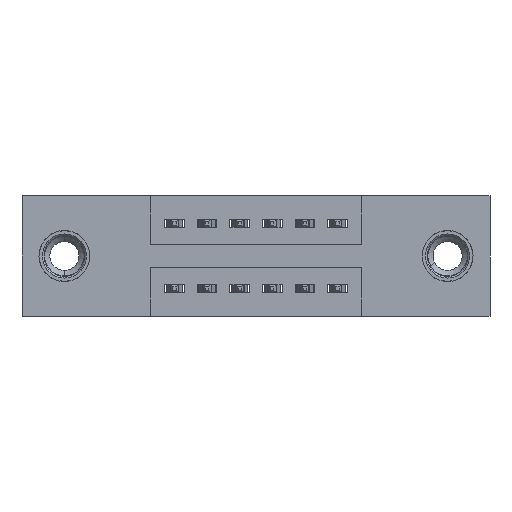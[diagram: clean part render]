
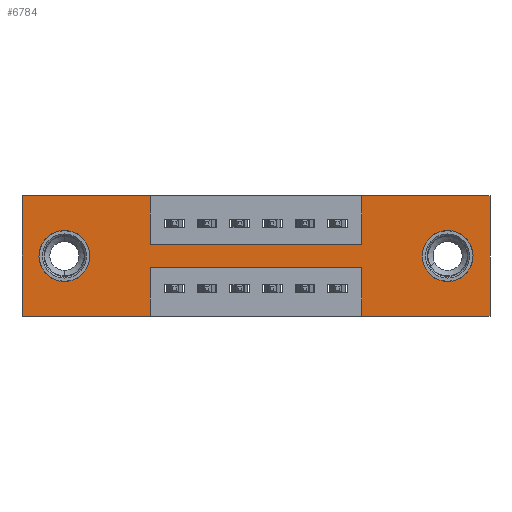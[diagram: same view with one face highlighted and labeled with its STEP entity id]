
A CAD part, front view. The second image highlights one B-rep face of the part: STEP entity #6784.
In plain terms, the highlighted planar face has unit normal (0, -1, 0).
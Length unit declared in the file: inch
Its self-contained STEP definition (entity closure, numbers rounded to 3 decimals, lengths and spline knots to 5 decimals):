
#75 = VERTEX_POINT ( 'NONE', #1648 ) ;
#120 = CARTESIAN_POINT ( 'NONE',  ( 0.13, 0., -0.185 ) ) ;
#124 = EDGE_CURVE ( 'NONE', #5131, #75, #7524, .T. ) ;
#136 = ORIENTED_EDGE ( 'NONE', *, *, #10163, .F. ) ;
#171 = VECTOR ( 'NONE', #3148, 39.37008 ) ;
#294 = LINE ( 'NONE', #9410, #8684 ) ;
#485 = DIRECTION ( 'NONE',  ( 1., 0., 0. ) ) ;
#491 = LINE ( 'NONE', #7586, #4763 ) ;
#546 = EDGE_CURVE ( 'NONE', #9718, #7218, #10677, .T. ) ;
#594 = VERTEX_POINT ( 'NONE', #8205 ) ;
#686 = AXIS2_PLACEMENT_3D ( 'NONE', #10744, #5892, #879 ) ;
#742 = EDGE_CURVE ( 'NONE', #75, #2618, #294, .T. ) ;
#811 = AXIS2_PLACEMENT_3D ( 'NONE', #6003, #996, #6815 ) ;
#876 = CIRCLE ( 'NONE', #9910, 0.078 ) ;
#879 = DIRECTION ( 'NONE',  ( 0., 0., 1. ) ) ;
#885 = PLANE ( 'NONE',  #5224 ) ;
#996 = DIRECTION ( 'NONE',  ( 0., 1., 0. ) ) ;
#1025 = DIRECTION ( 'NONE',  ( 0., 0., -1. ) ) ;
#1043 = DIRECTION ( 'NONE',  ( 0., 0., 1. ) ) ;
#1084 = CARTESIAN_POINT ( 'NONE',  ( 1.305, 0., -0.107 ) ) ;
#1213 = CARTESIAN_POINT ( 'NONE',  ( 0.3925, 0., 0. ) ) ;
#1319 = VERTEX_POINT ( 'NONE', #9587 ) ;
#1353 = EDGE_CURVE ( 'NONE', #5016, #7553, #8397, .T. ) ;
#1615 = VERTEX_POINT ( 'NONE', #6259 ) ;
#1645 = CARTESIAN_POINT ( 'NONE',  ( 1.0425, 0., 0. ) ) ;
#1648 = CARTESIAN_POINT ( 'NONE',  ( 0.3925, 0., -0.22 ) ) ;
#1689 = ORIENTED_EDGE ( 'NONE', *, *, #124, .F. ) ;
#1775 = DIRECTION ( 'NONE',  ( 0., 0., -1. ) ) ;
#1979 = VERTEX_POINT ( 'NONE', #8254 ) ;
#2053 = CARTESIAN_POINT ( 'NONE',  ( 1.305, 0., -0.263 ) ) ;
#2247 = ORIENTED_EDGE ( 'NONE', *, *, #9821, .F. ) ;
#2309 = VERTEX_POINT ( 'NONE', #7028 ) ;
#2618 = VERTEX_POINT ( 'NONE', #3358 ) ;
#2709 = CARTESIAN_POINT ( 'NONE',  ( 0.3925, 0., -0.15 ) ) ;
#2871 = FACE_BOUND ( 'NONE', #10533, .T. ) ;
#3089 = EDGE_LOOP ( 'NONE', ( #9894, #5834 ) ) ;
#3137 = ORIENTED_EDGE ( 'NONE', *, *, #1353, .T. ) ;
#3148 = DIRECTION ( 'NONE',  ( -1., 0., 0. ) ) ;
#3164 = VERTEX_POINT ( 'NONE', #8344 ) ;
#3282 = CARTESIAN_POINT ( 'NONE',  ( 1.435, 0., 0. ) ) ;
#3358 = CARTESIAN_POINT ( 'NONE',  ( 0.3925, 0., -0.37 ) ) ;
#3360 = CARTESIAN_POINT ( 'NONE',  ( 0.3925, 0., -0.22 ) ) ;
#3452 = EDGE_CURVE ( 'NONE', #1319, #3164, #8162, .T. ) ;
#3631 = EDGE_CURVE ( 'NONE', #2618, #2309, #4732, .T. ) ;
#3648 = CARTESIAN_POINT ( 'NONE',  ( 0.3925, 0., -0.15 ) ) ;
#3752 = VECTOR ( 'NONE', #9447, 39.37008 ) ;
#4158 = ORIENTED_EDGE ( 'NONE', *, *, #7450, .F. ) ;
#4180 = DIRECTION ( 'NONE',  ( 0., 0., -1. ) ) ;
#4237 = EDGE_LOOP ( 'NONE', ( #8005, #1689, #6103, #8256, #4158, #10658, #2247, #4429, #6604, #8795, #136, #4700 ) ) ;
#4297 = CARTESIAN_POINT ( 'NONE',  ( 1.305, 0., -0.185 ) ) ;
#4429 = ORIENTED_EDGE ( 'NONE', *, *, #9304, .F. ) ;
#4479 = EDGE_CURVE ( 'NONE', #1615, #1979, #5351, .T. ) ;
#4559 = VERTEX_POINT ( 'NONE', #2709 ) ;
#4600 = AXIS2_PLACEMENT_3D ( 'NONE', #4297, #8379, #8233 ) ;
#4700 = ORIENTED_EDGE ( 'NONE', *, *, #3631, .F. ) ;
#4732 = LINE ( 'NONE', #4815, #171 ) ;
#4763 = VECTOR ( 'NONE', #9213, 39.37008 ) ;
#4815 = CARTESIAN_POINT ( 'NONE',  ( 0., 0., -0.37 ) ) ;
#4956 = EDGE_CURVE ( 'NONE', #1979, #1615, #876, .T. ) ;
#5016 = VERTEX_POINT ( 'NONE', #1084 ) ;
#5131 = VERTEX_POINT ( 'NONE', #9504 ) ;
#5224 = AXIS2_PLACEMENT_3D ( 'NONE', #9161, #6718, #1775 ) ;
#5299 = FACE_BOUND ( 'NONE', #3089, .T. ) ;
#5351 = CIRCLE ( 'NONE', #686, 0.078 ) ;
#5354 = VECTOR ( 'NONE', #9142, 39.37008 ) ;
#5371 = CIRCLE ( 'NONE', #811, 0.078 ) ;
#5449 = CARTESIAN_POINT ( 'NONE',  ( 0., 0., 0. ) ) ;
#5580 = LINE ( 'NONE', #8760, #9655 ) ;
#5808 = EDGE_CURVE ( 'NONE', #8978, #594, #5580, .T. ) ;
#5834 = ORIENTED_EDGE ( 'NONE', *, *, #4479, .T. ) ;
#5892 = DIRECTION ( 'NONE',  ( 0., 1., 0. ) ) ;
#5998 = VECTOR ( 'NONE', #6279, 39.37008 ) ;
#6003 = CARTESIAN_POINT ( 'NONE',  ( 1.305, 0., -0.185 ) ) ;
#6019 = VECTOR ( 'NONE', #9645, 39.37008 ) ;
#6053 = DIRECTION ( 'NONE',  ( 0., 1., 0. ) ) ;
#6103 = ORIENTED_EDGE ( 'NONE', *, *, #10363, .F. ) ;
#6259 = CARTESIAN_POINT ( 'NONE',  ( 0.13, 0., -0.263 ) ) ;
#6279 = DIRECTION ( 'NONE',  ( 1., 0., 0. ) ) ;
#6411 = CARTESIAN_POINT ( 'NONE',  ( 0., 0., 0. ) ) ;
#6604 = ORIENTED_EDGE ( 'NONE', *, *, #8197, .F. ) ;
#6660 = VECTOR ( 'NONE', #10683, 39.37008 ) ;
#6718 = DIRECTION ( 'NONE',  ( 0., -1., 0. ) ) ;
#6784 = ADVANCED_FACE ( 'NONE', ( #2871, #5299, #6946 ), #885, .T. ) ;
#6815 = DIRECTION ( 'NONE',  ( 0., 0., -1. ) ) ;
#6842 = CARTESIAN_POINT ( 'NONE',  ( 1.435, 0., 0. ) ) ;
#6946 = FACE_OUTER_BOUND ( 'NONE', #4237, .T. ) ;
#7028 = CARTESIAN_POINT ( 'NONE',  ( 0., 0., -0.37 ) ) ;
#7218 = VERTEX_POINT ( 'NONE', #3282 ) ;
#7409 = VECTOR ( 'NONE', #8497, 39.37008 ) ;
#7450 = EDGE_CURVE ( 'NONE', #7218, #8978, #8486, .T. ) ;
#7524 = LINE ( 'NONE', #3360, #5354 ) ;
#7553 = VERTEX_POINT ( 'NONE', #2053 ) ;
#7586 = CARTESIAN_POINT ( 'NONE',  ( 1.0425, 0., 0. ) ) ;
#7749 = ORIENTED_EDGE ( 'NONE', *, *, #10464, .T. ) ;
#7830 = LINE ( 'NONE', #1213, #3752 ) ;
#8005 = ORIENTED_EDGE ( 'NONE', *, *, #742, .F. ) ;
#8162 = LINE ( 'NONE', #5449, #5998 ) ;
#8197 = EDGE_CURVE ( 'NONE', #3164, #4559, #7830, .T. ) ;
#8205 = CARTESIAN_POINT ( 'NONE',  ( 1.0425, 0., -0.37 ) ) ;
#8233 = DIRECTION ( 'NONE',  ( 0., 0., -1. ) ) ;
#8254 = CARTESIAN_POINT ( 'NONE',  ( 0.13, 0., -0.107 ) ) ;
#8256 = ORIENTED_EDGE ( 'NONE', *, *, #5808, .F. ) ;
#8288 = CARTESIAN_POINT ( 'NONE',  ( 1.0425, 0., -0.37 ) ) ;
#8344 = CARTESIAN_POINT ( 'NONE',  ( 0.3925, 0., 0. ) ) ;
#8379 = DIRECTION ( 'NONE',  ( 0., 1., 0. ) ) ;
#8397 = CIRCLE ( 'NONE', #4600, 0.078 ) ;
#8486 = LINE ( 'NONE', #6842, #10619 ) ;
#8497 = DIRECTION ( 'NONE',  ( 1., 0., 0. ) ) ;
#8684 = VECTOR ( 'NONE', #4180, 39.37008 ) ;
#8760 = CARTESIAN_POINT ( 'NONE',  ( 0., 0., -0.37 ) ) ;
#8795 = ORIENTED_EDGE ( 'NONE', *, *, #3452, .F. ) ;
#8938 = CARTESIAN_POINT ( 'NONE',  ( 1.435, 0., -0.37 ) ) ;
#8972 = LINE ( 'NONE', #6411, #6019 ) ;
#8978 = VERTEX_POINT ( 'NONE', #8938 ) ;
#9142 = DIRECTION ( 'NONE',  ( -1., 0., 0. ) ) ;
#9161 = CARTESIAN_POINT ( 'NONE',  ( 0., 0., -0.37 ) ) ;
#9213 = DIRECTION ( 'NONE',  ( 0., 0., 1. ) ) ;
#9275 = CARTESIAN_POINT ( 'NONE',  ( 1.0425, 0., -0.15 ) ) ;
#9304 = EDGE_CURVE ( 'NONE', #4559, #9857, #9585, .T. ) ;
#9410 = CARTESIAN_POINT ( 'NONE',  ( 0.3925, 0., -0.37 ) ) ;
#9447 = DIRECTION ( 'NONE',  ( 0., 0., -1. ) ) ;
#9504 = CARTESIAN_POINT ( 'NONE',  ( 1.0425, 0., -0.22 ) ) ;
#9553 = DIRECTION ( 'NONE',  ( -1., 0., 0. ) ) ;
#9585 = LINE ( 'NONE', #3648, #7409 ) ;
#9587 = CARTESIAN_POINT ( 'NONE',  ( 0., 0., 0. ) ) ;
#9645 = DIRECTION ( 'NONE',  ( 0., 0., 1. ) ) ;
#9655 = VECTOR ( 'NONE', #9553, 39.37008 ) ;
#9718 = VERTEX_POINT ( 'NONE', #1645 ) ;
#9821 = EDGE_CURVE ( 'NONE', #9857, #9718, #491, .T. ) ;
#9857 = VERTEX_POINT ( 'NONE', #9275 ) ;
#9873 = CARTESIAN_POINT ( 'NONE',  ( 0., 0., 0. ) ) ;
#9894 = ORIENTED_EDGE ( 'NONE', *, *, #4956, .T. ) ;
#9910 = AXIS2_PLACEMENT_3D ( 'NONE', #120, #6053, #1043 ) ;
#10163 = EDGE_CURVE ( 'NONE', #2309, #1319, #8972, .T. ) ;
#10179 = VECTOR ( 'NONE', #485, 39.37008 ) ;
#10363 = EDGE_CURVE ( 'NONE', #594, #5131, #10451, .T. ) ;
#10451 = LINE ( 'NONE', #8288, #6660 ) ;
#10464 = EDGE_CURVE ( 'NONE', #7553, #5016, #5371, .T. ) ;
#10533 = EDGE_LOOP ( 'NONE', ( #3137, #7749 ) ) ;
#10619 = VECTOR ( 'NONE', #1025, 39.37008 ) ;
#10658 = ORIENTED_EDGE ( 'NONE', *, *, #546, .F. ) ;
#10677 = LINE ( 'NONE', #9873, #10179 ) ;
#10683 = DIRECTION ( 'NONE',  ( 0., 0., 1. ) ) ;
#10744 = CARTESIAN_POINT ( 'NONE',  ( 0.13, 0., -0.185 ) ) ;
